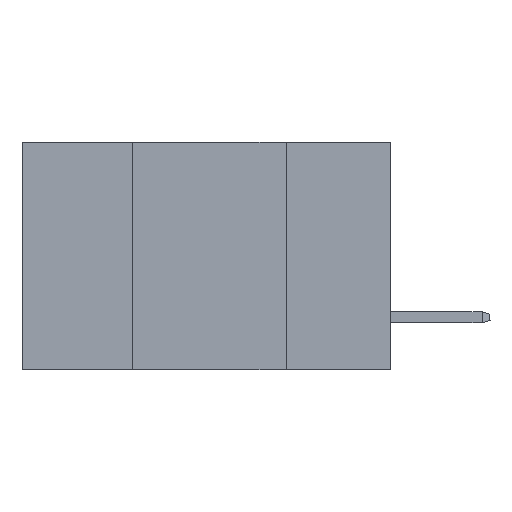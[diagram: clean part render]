
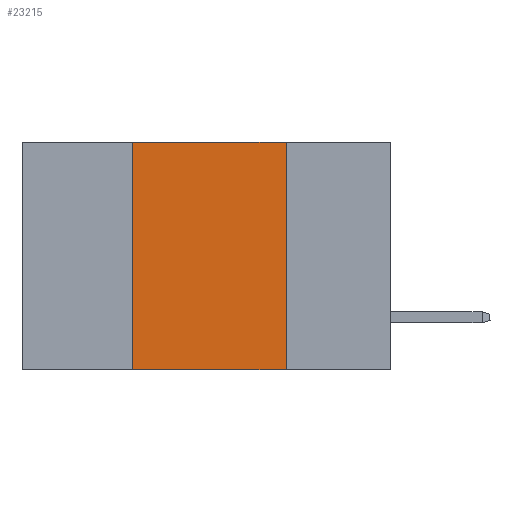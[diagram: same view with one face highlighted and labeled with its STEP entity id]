
A CAD part, left-side view. The second image highlights one B-rep face of the part: STEP entity #23215.
In plain terms, the highlighted planar face has unit normal (-1, 0, 0).
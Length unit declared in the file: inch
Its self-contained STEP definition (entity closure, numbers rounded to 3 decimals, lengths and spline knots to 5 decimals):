
#386 = ORIENTED_EDGE ( 'NONE', *, *, #16298, .F. ) ;
#470 = DIRECTION ( 'NONE',  ( 0., 0., -1. ) ) ;
#3653 = EDGE_CURVE ( 'NONE', #22019, #38208, #32274, .T. ) ;
#3825 = CARTESIAN_POINT ( 'NONE',  ( 0., 0.42, 0. ) ) ;
#4374 = CARTESIAN_POINT ( 'NONE',  ( 0., 0.6, -0.37 ) ) ;
#4712 = VECTOR ( 'NONE', #4860, 39.37008 ) ;
#4860 = DIRECTION ( 'NONE',  ( 0., -1., 0. ) ) ;
#9898 = DIRECTION ( 'NONE',  ( 0., 0., -1. ) ) ;
#16202 = VERTEX_POINT ( 'NONE', #18098 ) ;
#16298 = EDGE_CURVE ( 'NONE', #38351, #16202, #17982, .T. ) ;
#17211 = CARTESIAN_POINT ( 'NONE',  ( 0., 0.17, 0. ) ) ;
#17456 = CARTESIAN_POINT ( 'NONE',  ( 0., 0.6, 0. ) ) ;
#17982 = LINE ( 'NONE', #3825, #32033 ) ;
#18098 = CARTESIAN_POINT ( 'NONE',  ( 0., 0.42, 0. ) ) ;
#18438 = DIRECTION ( 'NONE',  ( 0., 0., 1. ) ) ;
#18779 = AXIS2_PLACEMENT_3D ( 'NONE', #45390, #41607, #470 ) ;
#22019 = VERTEX_POINT ( 'NONE', #17211 ) ;
#22304 = EDGE_CURVE ( 'NONE', #16202, #22019, #26123, .T. ) ;
#23215 = ADVANCED_FACE ( 'NONE', ( #24246 ), #37497, .F. ) ;
#24246 = FACE_OUTER_BOUND ( 'NONE', #42155, .T. ) ;
#26123 = LINE ( 'NONE', #17456, #40189 ) ;
#26419 = ORIENTED_EDGE ( 'NONE', *, *, #47052, .T. ) ;
#28137 = LINE ( 'NONE', #4374, #4712 ) ;
#28392 = DIRECTION ( 'NONE',  ( 0., -1., 0. ) ) ;
#30706 = CARTESIAN_POINT ( 'NONE',  ( 0., 0.17, -0.37 ) ) ;
#32033 = VECTOR ( 'NONE', #18438, 39.37008 ) ;
#32274 = LINE ( 'NONE', #44163, #35803 ) ;
#35803 = VECTOR ( 'NONE', #9898, 39.37008 ) ;
#37497 = PLANE ( 'NONE',  #18779 ) ;
#38208 = VERTEX_POINT ( 'NONE', #30706 ) ;
#38351 = VERTEX_POINT ( 'NONE', #39254 ) ;
#39254 = CARTESIAN_POINT ( 'NONE',  ( 0., 0.42, -0.37 ) ) ;
#40189 = VECTOR ( 'NONE', #28392, 39.37008 ) ;
#41607 = DIRECTION ( 'NONE',  ( 1., 0., 0. ) ) ;
#42155 = EDGE_LOOP ( 'NONE', ( #46218, #47852, #386, #26419 ) ) ;
#44163 = CARTESIAN_POINT ( 'NONE',  ( 0., 0.17, 0. ) ) ;
#45390 = CARTESIAN_POINT ( 'NONE',  ( 0., 0.6, 0. ) ) ;
#46218 = ORIENTED_EDGE ( 'NONE', *, *, #3653, .F. ) ;
#47052 = EDGE_CURVE ( 'NONE', #38351, #38208, #28137, .T. ) ;
#47852 = ORIENTED_EDGE ( 'NONE', *, *, #22304, .F. ) ;
